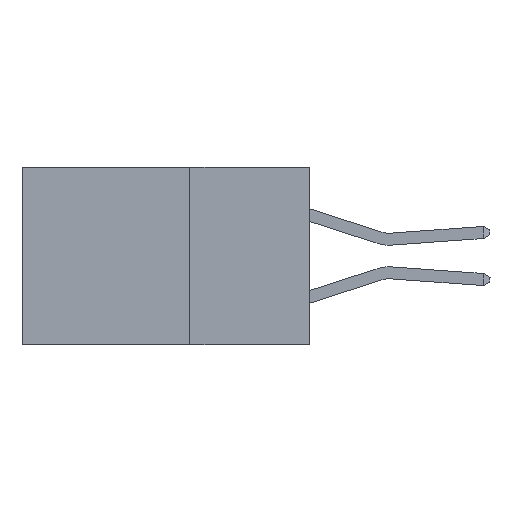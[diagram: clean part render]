
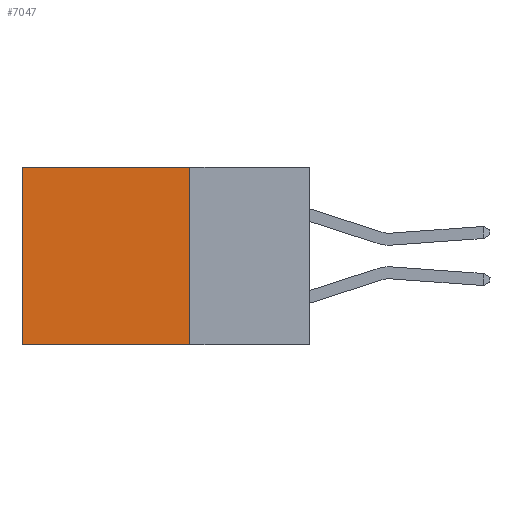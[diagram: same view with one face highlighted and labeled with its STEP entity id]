
A CAD part, left-side view. The second image highlights one B-rep face of the part: STEP entity #7047.
In plain terms, the highlighted planar face has unit normal (-1, 0, 0).
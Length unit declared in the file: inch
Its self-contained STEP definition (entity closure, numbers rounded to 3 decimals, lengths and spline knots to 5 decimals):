
#19 = CARTESIAN_POINT ( 'NONE',  ( 0.2615, 0.25, -0.37 ) ) ;
#728 = DIRECTION ( 'NONE',  ( 0., 0., -1. ) ) ;
#1176 = DIRECTION ( 'NONE',  ( 0., 0., -1. ) ) ;
#1247 = VERTEX_POINT ( 'NONE', #7555 ) ;
#1401 = EDGE_CURVE ( 'NONE', #1247, #5979, #2756, .T. ) ;
#1494 = VERTEX_POINT ( 'NONE', #3324 ) ;
#1518 = ORIENTED_EDGE ( 'NONE', *, *, #6226, .T. ) ;
#1765 = PLANE ( 'NONE',  #7401 ) ;
#2415 = LINE ( 'NONE', #8186, #7287 ) ;
#2511 = VECTOR ( 'NONE', #8584, 39.37008 ) ;
#2756 = LINE ( 'NONE', #19, #2511 ) ;
#3016 = FACE_OUTER_BOUND ( 'NONE', #7175, .T. ) ;
#3169 = LINE ( 'NONE', #7436, #7669 ) ;
#3324 = CARTESIAN_POINT ( 'NONE',  ( 0.2615, 0.25, 0. ) ) ;
#3358 = CARTESIAN_POINT ( 'NONE',  ( 0.2615, 0.25, -0.37 ) ) ;
#3581 = ORIENTED_EDGE ( 'NONE', *, *, #1401, .F. ) ;
#4013 = DIRECTION ( 'NONE',  ( 0., 0., -1. ) ) ;
#4720 = VECTOR ( 'NONE', #728, 39.37008 ) ;
#5012 = ORIENTED_EDGE ( 'NONE', *, *, #9926, .F. ) ;
#5073 = EDGE_CURVE ( 'NONE', #5342, #5979, #3169, .T. ) ;
#5342 = VERTEX_POINT ( 'NONE', #5492 ) ;
#5492 = CARTESIAN_POINT ( 'NONE',  ( 0.2615, 0.6, 0. ) ) ;
#5979 = VERTEX_POINT ( 'NONE', #6161 ) ;
#6161 = CARTESIAN_POINT ( 'NONE',  ( 0.2615, 0.6, -0.37 ) ) ;
#6226 = EDGE_CURVE ( 'NONE', #1494, #5342, #2415, .T. ) ;
#6373 = DIRECTION ( 'NONE',  ( 1., 0., 0. ) ) ;
#7047 = ADVANCED_FACE ( 'NONE', ( #3016 ), #1765, .F. ) ;
#7175 = EDGE_LOOP ( 'NONE', ( #9845, #3581, #5012, #1518 ) ) ;
#7287 = VECTOR ( 'NONE', #9790, 39.37008 ) ;
#7401 = AXIS2_PLACEMENT_3D ( 'NONE', #3358, #6373, #4013 ) ;
#7436 = CARTESIAN_POINT ( 'NONE',  ( 0.2615, 0.6, -0.37 ) ) ;
#7555 = CARTESIAN_POINT ( 'NONE',  ( 0.2615, 0.25, -0.37 ) ) ;
#7669 = VECTOR ( 'NONE', #1176, 39.37008 ) ;
#8186 = CARTESIAN_POINT ( 'NONE',  ( 0.2615, 0.25, 0. ) ) ;
#8584 = DIRECTION ( 'NONE',  ( 0., 1., 0. ) ) ;
#9790 = DIRECTION ( 'NONE',  ( 0., 1., 0. ) ) ;
#9845 = ORIENTED_EDGE ( 'NONE', *, *, #5073, .T. ) ;
#9926 = EDGE_CURVE ( 'NONE', #1494, #1247, #10071, .T. ) ;
#10071 = LINE ( 'NONE', #10114, #4720 ) ;
#10114 = CARTESIAN_POINT ( 'NONE',  ( 0.2615, 0.25, -0.37 ) ) ;
